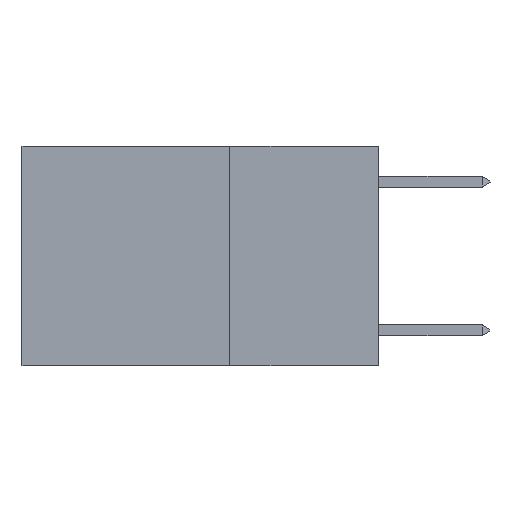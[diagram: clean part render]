
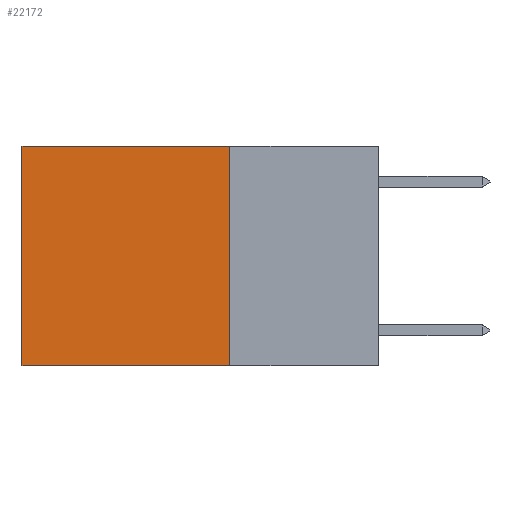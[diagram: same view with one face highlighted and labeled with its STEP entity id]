
A CAD part, left-side view. The second image highlights one B-rep face of the part: STEP entity #22172.
In plain terms, the highlighted planar face has unit normal (-1, 0, 0).
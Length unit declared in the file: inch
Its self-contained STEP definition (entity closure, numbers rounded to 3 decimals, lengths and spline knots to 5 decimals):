
#1596 = ORIENTED_EDGE ( 'NONE', *, *, #7711, .F. ) ;
#2318 = EDGE_CURVE ( 'NONE', #20661, #21993, #9457, .T. ) ;
#2587 = VECTOR ( 'NONE', #18622, 39.37008 ) ;
#4265 = DIRECTION ( 'NONE',  ( 1., 0., 0. ) ) ;
#4518 = VERTEX_POINT ( 'NONE', #18322 ) ;
#7574 = DIRECTION ( 'NONE',  ( 0., 0., -1. ) ) ;
#7711 = EDGE_CURVE ( 'NONE', #4518, #21993, #8965, .T. ) ;
#7746 = EDGE_CURVE ( 'NONE', #13979, #4518, #22298, .T. ) ;
#8078 = ORIENTED_EDGE ( 'NONE', *, *, #2318, .T. ) ;
#8965 = LINE ( 'NONE', #20660, #2587 ) ;
#9457 = LINE ( 'NONE', #17115, #9754 ) ;
#9754 = VECTOR ( 'NONE', #7574, 39.37008 ) ;
#10682 = VECTOR ( 'NONE', #12624, 39.37008 ) ;
#10739 = CARTESIAN_POINT ( 'NONE',  ( 0.2625, 0.25, 0. ) ) ;
#12192 = LINE ( 'NONE', #12315, #14231 ) ;
#12315 = CARTESIAN_POINT ( 'NONE',  ( 0.2625, 0.25, 0. ) ) ;
#12624 = DIRECTION ( 'NONE',  ( 0., 0., -1. ) ) ;
#12856 = EDGE_LOOP ( 'NONE', ( #8078, #1596, #19425, #22377 ) ) ;
#13147 = EDGE_CURVE ( 'NONE', #13979, #20661, #12192, .T. ) ;
#13979 = VERTEX_POINT ( 'NONE', #21429 ) ;
#14231 = VECTOR ( 'NONE', #19959, 39.37008 ) ;
#16059 = CARTESIAN_POINT ( 'NONE',  ( 0.2625, 0.25, 0. ) ) ;
#17115 = CARTESIAN_POINT ( 'NONE',  ( 0.2625, 0.6, 0. ) ) ;
#18322 = CARTESIAN_POINT ( 'NONE',  ( 0.2625, 0.25, -0.37 ) ) ;
#18622 = DIRECTION ( 'NONE',  ( 0., 1., 0. ) ) ;
#19213 = CARTESIAN_POINT ( 'NONE',  ( 0.2625, 0.6, -0.37 ) ) ;
#19425 = ORIENTED_EDGE ( 'NONE', *, *, #7746, .F. ) ;
#19558 = CARTESIAN_POINT ( 'NONE',  ( 0.2625, 0.6, 0. ) ) ;
#19854 = PLANE ( 'NONE',  #21723 ) ;
#19959 = DIRECTION ( 'NONE',  ( 0., 1., 0. ) ) ;
#20660 = CARTESIAN_POINT ( 'NONE',  ( 0.2625, 0.25, -0.37 ) ) ;
#20661 = VERTEX_POINT ( 'NONE', #19558 ) ;
#21429 = CARTESIAN_POINT ( 'NONE',  ( 0.2625, 0.25, 0. ) ) ;
#21506 = FACE_OUTER_BOUND ( 'NONE', #12856, .T. ) ;
#21723 = AXIS2_PLACEMENT_3D ( 'NONE', #16059, #4265, #23757 ) ;
#21993 = VERTEX_POINT ( 'NONE', #19213 ) ;
#22172 = ADVANCED_FACE ( 'NONE', ( #21506 ), #19854, .F. ) ;
#22298 = LINE ( 'NONE', #10739, #10682 ) ;
#22377 = ORIENTED_EDGE ( 'NONE', *, *, #13147, .T. ) ;
#23757 = DIRECTION ( 'NONE',  ( 0., 0., -1. ) ) ;
